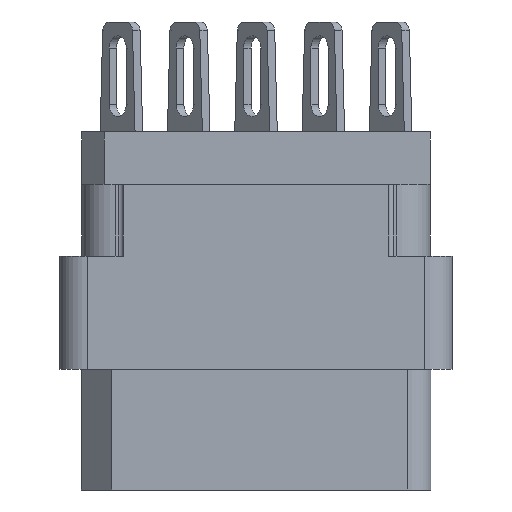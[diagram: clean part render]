
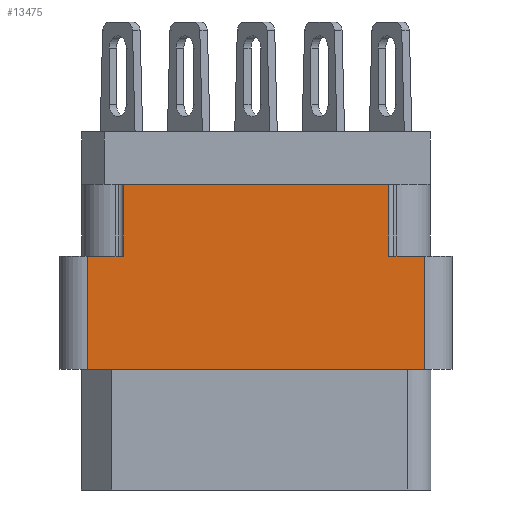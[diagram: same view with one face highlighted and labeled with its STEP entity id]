
A CAD part, left-side view. The second image highlights one B-rep face of the part: STEP entity #13475.
In plain terms, the highlighted planar face has unit normal (-1, 0, 0).
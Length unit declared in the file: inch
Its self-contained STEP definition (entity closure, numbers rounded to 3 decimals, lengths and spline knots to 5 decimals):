
#562 = LINE ( 'NONE', #10544, #21480 ) ;
#964 = EDGE_CURVE ( 'NONE', #10522, #17422, #31732, .T. ) ;
#1630 = VERTEX_POINT ( 'NONE', #20972 ) ;
#1781 = VECTOR ( 'NONE', #21642, 39.37008 ) ;
#3597 = LINE ( 'NONE', #16413, #8061 ) ;
#3943 = EDGE_CURVE ( 'NONE', #22985, #17422, #21128, .T. ) ;
#4270 = AXIS2_PLACEMENT_3D ( 'NONE', #25263, #32312, #10144 ) ;
#4567 = CARTESIAN_POINT ( 'NONE',  ( -1., -0.376, -0.529 ) ) ;
#5227 = FACE_OUTER_BOUND ( 'NONE', #12382, .T. ) ;
#6102 = ORIENTED_EDGE ( 'NONE', *, *, #26734, .F. ) ;
#6927 = DIRECTION ( 'NONE',  ( 0., 0., 1. ) ) ;
#8061 = VECTOR ( 'NONE', #10830, 39.37008 ) ;
#8819 = EDGE_CURVE ( 'NONE', #10522, #12042, #3597, .T. ) ;
#9247 = DIRECTION ( 'NONE',  ( 0., 0., 1. ) ) ;
#9318 = LINE ( 'NONE', #4567, #1781 ) ;
#9931 = ORIENTED_EDGE ( 'NONE', *, *, #10080, .F. ) ;
#10080 = EDGE_CURVE ( 'NONE', #13091, #18001, #562, .T. ) ;
#10144 = DIRECTION ( 'NONE',  ( 0., 0., 1. ) ) ;
#10522 = VERTEX_POINT ( 'NONE', #27913 ) ;
#10544 = CARTESIAN_POINT ( 'NONE',  ( -1., 0.376, -0.798 ) ) ;
#10830 = DIRECTION ( 'NONE',  ( 0., -1., 0. ) ) ;
#11774 = VECTOR ( 'NONE', #25571, 39.37008 ) ;
#12042 = VERTEX_POINT ( 'NONE', #30515 ) ;
#12382 = EDGE_LOOP ( 'NONE', ( #9931, #25598, #30083, #18910, #17903, #14306, #6102, #21379 ) ) ;
#12892 = VECTOR ( 'NONE', #9247, 39.37008 ) ;
#13091 = VERTEX_POINT ( 'NONE', #19613 ) ;
#13234 = CARTESIAN_POINT ( 'NONE',  ( -1., 0.296, -0.277 ) ) ;
#13475 = ADVANCED_FACE ( 'NONE', ( #5227 ), #20186, .T. ) ;
#14306 = ORIENTED_EDGE ( 'NONE', *, *, #3943, .F. ) ;
#14344 = CARTESIAN_POINT ( 'NONE',  ( -1., -0.296, -0.277 ) ) ;
#15819 = VECTOR ( 'NONE', #6927, 39.37008 ) ;
#15902 = EDGE_CURVE ( 'NONE', #27412, #13091, #9318, .T. ) ;
#16413 = CARTESIAN_POINT ( 'NONE',  ( -1., -0.296, -0.277 ) ) ;
#17119 = VECTOR ( 'NONE', #25556, 39.37008 ) ;
#17422 = VERTEX_POINT ( 'NONE', #27581 ) ;
#17903 = ORIENTED_EDGE ( 'NONE', *, *, #964, .T. ) ;
#18001 = VERTEX_POINT ( 'NONE', #28927 ) ;
#18064 = LINE ( 'NONE', #30663, #21874 ) ;
#18291 = DIRECTION ( 'NONE',  ( 0., 0., 1. ) ) ;
#18910 = ORIENTED_EDGE ( 'NONE', *, *, #8819, .F. ) ;
#19430 = LINE ( 'NONE', #29393, #15819 ) ;
#19613 = CARTESIAN_POINT ( 'NONE',  ( -1., 0.376, -0.529 ) ) ;
#20186 = PLANE ( 'NONE',  #4270 ) ;
#20202 = CARTESIAN_POINT ( 'NONE',  ( -1., -0.376, -0.529 ) ) ;
#20651 = CARTESIAN_POINT ( 'NONE',  ( -1., 0.438, -0.117 ) ) ;
#20878 = EDGE_CURVE ( 'NONE', #27412, #12042, #19430, .T. ) ;
#20972 = CARTESIAN_POINT ( 'NONE',  ( -1., 0.296, -0.277 ) ) ;
#21128 = LINE ( 'NONE', #20651, #11774 ) ;
#21379 = ORIENTED_EDGE ( 'NONE', *, *, #27644, .F. ) ;
#21480 = VECTOR ( 'NONE', #18291, 39.37008 ) ;
#21642 = DIRECTION ( 'NONE',  ( 0., 1., 0. ) ) ;
#21874 = VECTOR ( 'NONE', #28044, 39.37008 ) ;
#22941 = LINE ( 'NONE', #13234, #17119 ) ;
#22985 = VERTEX_POINT ( 'NONE', #27051 ) ;
#25263 = CARTESIAN_POINT ( 'NONE',  ( -1., -0.376, -0.798 ) ) ;
#25556 = DIRECTION ( 'NONE',  ( 0., 0., 1. ) ) ;
#25571 = DIRECTION ( 'NONE',  ( 0., -1., 0. ) ) ;
#25598 = ORIENTED_EDGE ( 'NONE', *, *, #15902, .F. ) ;
#26734 = EDGE_CURVE ( 'NONE', #1630, #22985, #22941, .T. ) ;
#27051 = CARTESIAN_POINT ( 'NONE',  ( -1., 0.296, -0.117 ) ) ;
#27412 = VERTEX_POINT ( 'NONE', #20202 ) ;
#27581 = CARTESIAN_POINT ( 'NONE',  ( -1., -0.296, -0.117 ) ) ;
#27644 = EDGE_CURVE ( 'NONE', #18001, #1630, #18064, .T. ) ;
#27913 = CARTESIAN_POINT ( 'NONE',  ( -1., -0.296, -0.277 ) ) ;
#28044 = DIRECTION ( 'NONE',  ( 0., -1., 0. ) ) ;
#28927 = CARTESIAN_POINT ( 'NONE',  ( -1., 0.376, -0.277 ) ) ;
#29393 = CARTESIAN_POINT ( 'NONE',  ( -1., -0.376, -0.798 ) ) ;
#30083 = ORIENTED_EDGE ( 'NONE', *, *, #20878, .T. ) ;
#30515 = CARTESIAN_POINT ( 'NONE',  ( -1., -0.376, -0.277 ) ) ;
#30663 = CARTESIAN_POINT ( 'NONE',  ( -1., 0.438, -0.277 ) ) ;
#31732 = LINE ( 'NONE', #14344, #12892 ) ;
#32312 = DIRECTION ( 'NONE',  ( -1., 0., 0. ) ) ;
